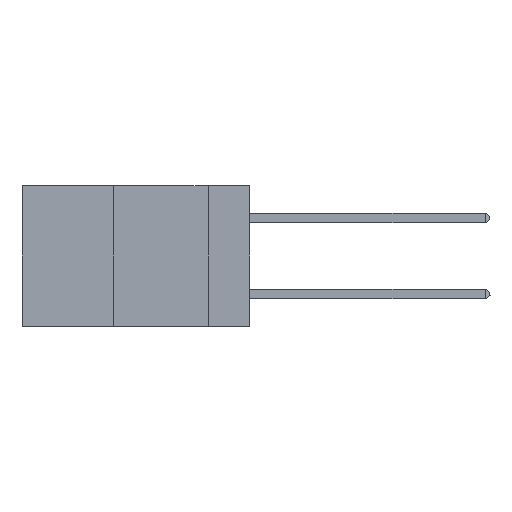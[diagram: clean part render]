
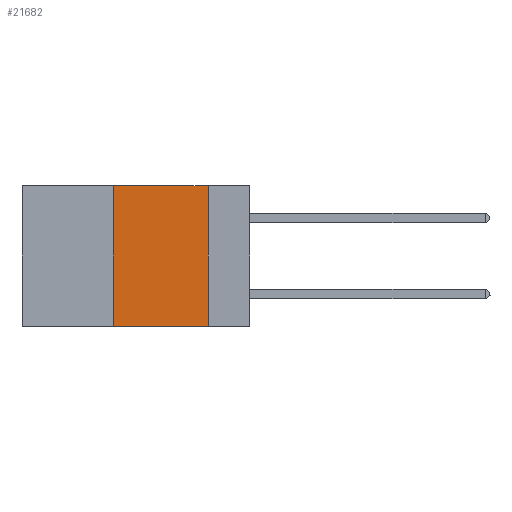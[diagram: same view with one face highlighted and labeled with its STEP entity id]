
A CAD part, left-side view. The second image highlights one B-rep face of the part: STEP entity #21682.
In plain terms, the highlighted planar face has unit normal (-1, 0, 0).
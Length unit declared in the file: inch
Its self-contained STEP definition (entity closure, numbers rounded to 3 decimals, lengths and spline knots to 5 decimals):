
#780 = CARTESIAN_POINT ( 'NONE',  ( 0., 0.36, -0.37 ) ) ;
#2065 = LINE ( 'NONE', #40217, #27109 ) ;
#2477 = EDGE_CURVE ( 'NONE', #34578, #2508, #23163, .T. ) ;
#2508 = VERTEX_POINT ( 'NONE', #34524 ) ;
#2796 = VECTOR ( 'NONE', #37779, 39.37008 ) ;
#5870 = EDGE_LOOP ( 'NONE', ( #40401, #11821, #37335, #23123 ) ) ;
#7835 = VECTOR ( 'NONE', #21178, 39.37008 ) ;
#11821 = ORIENTED_EDGE ( 'NONE', *, *, #35391, .F. ) ;
#12640 = VERTEX_POINT ( 'NONE', #39642 ) ;
#12681 = FACE_OUTER_BOUND ( 'NONE', #5870, .T. ) ;
#13014 = DIRECTION ( 'NONE',  ( 0., 0., -1. ) ) ;
#14018 = DIRECTION ( 'NONE',  ( 0., -1., 0. ) ) ;
#15895 = EDGE_CURVE ( 'NONE', #34578, #12640, #2065, .T. ) ;
#16270 = EDGE_CURVE ( 'NONE', #27181, #12640, #28585, .T. ) ;
#16846 = AXIS2_PLACEMENT_3D ( 'NONE', #24340, #17890, #33813 ) ;
#17855 = VECTOR ( 'NONE', #13014, 39.37008 ) ;
#17890 = DIRECTION ( 'NONE',  ( 1., 0., 0. ) ) ;
#20780 = PLANE ( 'NONE',  #16846 ) ;
#21178 = DIRECTION ( 'NONE',  ( 0., 0., 1. ) ) ;
#21682 = ADVANCED_FACE ( 'NONE', ( #12681 ), #20780, .F. ) ;
#23123 = ORIENTED_EDGE ( 'NONE', *, *, #15895, .T. ) ;
#23163 = LINE ( 'NONE', #30722, #7835 ) ;
#24340 = CARTESIAN_POINT ( 'NONE',  ( 0., 0.6, 0. ) ) ;
#27109 = VECTOR ( 'NONE', #14018, 39.37008 ) ;
#27181 = VERTEX_POINT ( 'NONE', #27958 ) ;
#27958 = CARTESIAN_POINT ( 'NONE',  ( 0., 0.11, 0. ) ) ;
#28585 = LINE ( 'NONE', #41346, #17855 ) ;
#30722 = CARTESIAN_POINT ( 'NONE',  ( 0., 0.36, 0. ) ) ;
#31897 = LINE ( 'NONE', #37354, #2796 ) ;
#33813 = DIRECTION ( 'NONE',  ( 0., 0., -1. ) ) ;
#34524 = CARTESIAN_POINT ( 'NONE',  ( 0., 0.36, 0. ) ) ;
#34578 = VERTEX_POINT ( 'NONE', #780 ) ;
#35391 = EDGE_CURVE ( 'NONE', #2508, #27181, #31897, .T. ) ;
#37335 = ORIENTED_EDGE ( 'NONE', *, *, #2477, .F. ) ;
#37354 = CARTESIAN_POINT ( 'NONE',  ( 0., 0.6, 0. ) ) ;
#37779 = DIRECTION ( 'NONE',  ( 0., -1., 0. ) ) ;
#39642 = CARTESIAN_POINT ( 'NONE',  ( 0., 0.11, -0.37 ) ) ;
#40217 = CARTESIAN_POINT ( 'NONE',  ( 0., 0.6, -0.37 ) ) ;
#40401 = ORIENTED_EDGE ( 'NONE', *, *, #16270, .F. ) ;
#41346 = CARTESIAN_POINT ( 'NONE',  ( 0., 0.11, 0. ) ) ;
